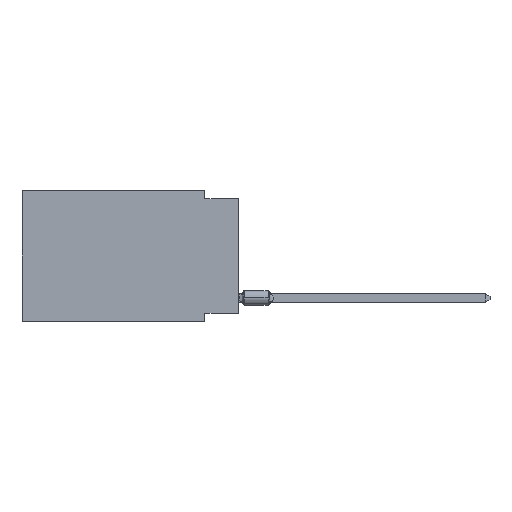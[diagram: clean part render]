
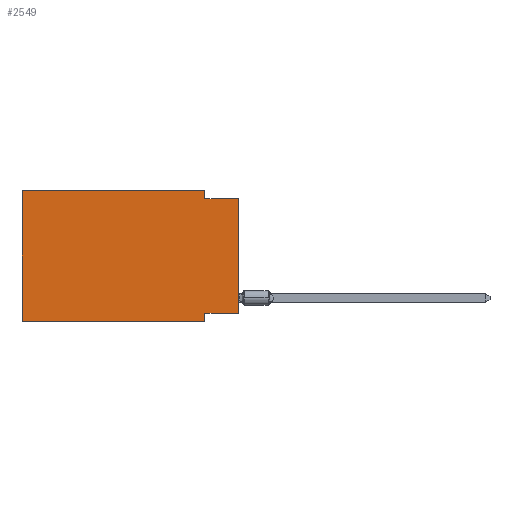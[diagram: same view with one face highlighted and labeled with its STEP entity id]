
A CAD part, left-side view. The second image highlights one B-rep face of the part: STEP entity #2549.
In plain terms, the highlighted planar face has unit normal (-1, 0, 0).
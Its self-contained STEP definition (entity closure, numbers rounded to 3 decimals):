
#412 = LINE ( 'NONE', #8796, #1270 ) ;
#618 = CARTESIAN_POINT ( 'NONE',  ( 0., 16.383, -9.906 ) ) ;
#697 = DIRECTION ( 'NONE',  ( 0., -1., 0. ) ) ;
#788 = CARTESIAN_POINT ( 'NONE',  ( 0., 16.383, -9.906 ) ) ;
#1115 = CARTESIAN_POINT ( 'NONE',  ( 0., 2.54, -9.906 ) ) ;
#1270 = VECTOR ( 'NONE', #7321, 1000. ) ;
#1552 = CARTESIAN_POINT ( 'NONE',  ( 0., 0., -0.635 ) ) ;
#1564 = VERTEX_POINT ( 'NONE', #8148 ) ;
#1760 = CARTESIAN_POINT ( 'NONE',  ( 0., 2.54, -9.906 ) ) ;
#2549 = ADVANCED_FACE ( 'NONE', ( #11593 ), #18721, .F. ) ;
#3300 = CARTESIAN_POINT ( 'NONE',  ( 0., 2.54, 0. ) ) ;
#3495 = DIRECTION ( 'NONE',  ( 0., 0., -1. ) ) ;
#3602 = CARTESIAN_POINT ( 'NONE',  ( 0., 0., -9.271 ) ) ;
#4096 = CARTESIAN_POINT ( 'NONE',  ( 0., 0., -0.635 ) ) ;
#4125 = LINE ( 'NONE', #618, #19604 ) ;
#4142 = EDGE_CURVE ( 'NONE', #17872, #18663, #13944, .T. ) ;
#4319 = EDGE_CURVE ( 'NONE', #18498, #10056, #9843, .T. ) ;
#5396 = ORIENTED_EDGE ( 'NONE', *, *, #18875, .F. ) ;
#5851 = CARTESIAN_POINT ( 'NONE',  ( 0., 16.383, 0. ) ) ;
#5882 = CARTESIAN_POINT ( 'NONE',  ( 0., 0., 0. ) ) ;
#6823 = VERTEX_POINT ( 'NONE', #12109 ) ;
#6962 = DIRECTION ( 'NONE',  ( 0., 0., -1. ) ) ;
#6979 = VECTOR ( 'NONE', #6962, 1000. ) ;
#7075 = VECTOR ( 'NONE', #20252, 1000. ) ;
#7164 = VERTEX_POINT ( 'NONE', #1115 ) ;
#7321 = DIRECTION ( 'NONE',  ( 0., 1., 0. ) ) ;
#7524 = DIRECTION ( 'NONE',  ( 0., -1., 0. ) ) ;
#8148 = CARTESIAN_POINT ( 'NONE',  ( 0., 2.54, -0.635 ) ) ;
#8654 = ORIENTED_EDGE ( 'NONE', *, *, #17261, .F. ) ;
#8796 = CARTESIAN_POINT ( 'NONE',  ( 0., 0., -9.271 ) ) ;
#9637 = DIRECTION ( 'NONE',  ( 0., 0., 1. ) ) ;
#9843 = LINE ( 'NONE', #13458, #7075 ) ;
#10056 = VERTEX_POINT ( 'NONE', #3300 ) ;
#10791 = LINE ( 'NONE', #4096, #12380 ) ;
#11284 = ORIENTED_EDGE ( 'NONE', *, *, #16823, .T. ) ;
#11301 = EDGE_CURVE ( 'NONE', #17872, #6823, #412, .T. ) ;
#11593 = FACE_OUTER_BOUND ( 'NONE', #20889, .T. ) ;
#11711 = CARTESIAN_POINT ( 'NONE',  ( 0., 16.383, 0. ) ) ;
#11984 = VECTOR ( 'NONE', #3495, 1000. ) ;
#12077 = CARTESIAN_POINT ( 'NONE',  ( 0., 16.383, 0. ) ) ;
#12109 = CARTESIAN_POINT ( 'NONE',  ( 0., 2.54, -9.271 ) ) ;
#12380 = VECTOR ( 'NONE', #697, 1000. ) ;
#13458 = CARTESIAN_POINT ( 'NONE',  ( 0., 16.383, 0. ) ) ;
#13944 = LINE ( 'NONE', #5882, #19009 ) ;
#13996 = DIRECTION ( 'NONE',  ( 0., 0., 1. ) ) ;
#14117 = ORIENTED_EDGE ( 'NONE', *, *, #4319, .F. ) ;
#15000 = DIRECTION ( 'NONE',  ( 1., 0., 0. ) ) ;
#15336 = ORIENTED_EDGE ( 'NONE', *, *, #11301, .F. ) ;
#15348 = AXIS2_PLACEMENT_3D ( 'NONE', #11711, #15000, #17017 ) ;
#15594 = EDGE_CURVE ( 'NONE', #6823, #7164, #17265, .T. ) ;
#16823 = EDGE_CURVE ( 'NONE', #19758, #7164, #4125, .T. ) ;
#17017 = DIRECTION ( 'NONE',  ( 0., 0., -1. ) ) ;
#17261 = EDGE_CURVE ( 'NONE', #1564, #18663, #10791, .T. ) ;
#17265 = LINE ( 'NONE', #1760, #6979 ) ;
#17682 = ORIENTED_EDGE ( 'NONE', *, *, #4142, .T. ) ;
#17872 = VERTEX_POINT ( 'NONE', #3602 ) ;
#18406 = ORIENTED_EDGE ( 'NONE', *, *, #21680, .F. ) ;
#18447 = VECTOR ( 'NONE', #13996, 1000. ) ;
#18498 = VERTEX_POINT ( 'NONE', #5851 ) ;
#18663 = VERTEX_POINT ( 'NONE', #1552 ) ;
#18721 = PLANE ( 'NONE',  #15348 ) ;
#18875 = EDGE_CURVE ( 'NONE', #19758, #18498, #19297, .T. ) ;
#18983 = LINE ( 'NONE', #22160, #11984 ) ;
#19009 = VECTOR ( 'NONE', #9637, 1000. ) ;
#19297 = LINE ( 'NONE', #12077, #18447 ) ;
#19604 = VECTOR ( 'NONE', #7524, 1000. ) ;
#19758 = VERTEX_POINT ( 'NONE', #788 ) ;
#20252 = DIRECTION ( 'NONE',  ( 0., -1., 0. ) ) ;
#20889 = EDGE_LOOP ( 'NONE', ( #17682, #8654, #18406, #14117, #5396, #11284, #20979, #15336 ) ) ;
#20979 = ORIENTED_EDGE ( 'NONE', *, *, #15594, .F. ) ;
#21680 = EDGE_CURVE ( 'NONE', #10056, #1564, #18983, .T. ) ;
#22160 = CARTESIAN_POINT ( 'NONE',  ( 0., 2.54, 0. ) ) ;
